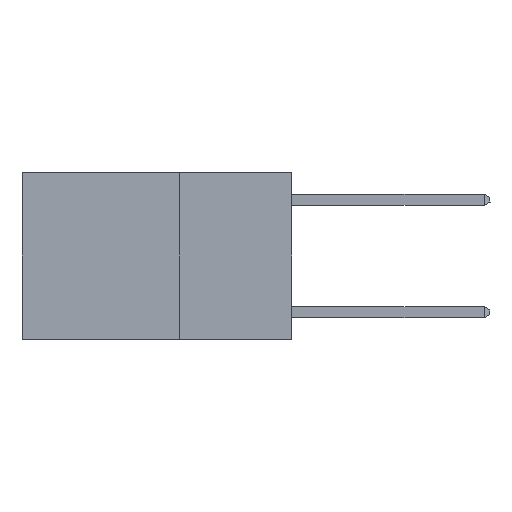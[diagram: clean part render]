
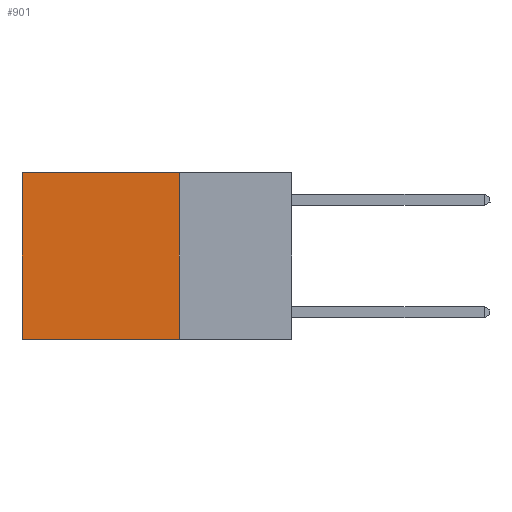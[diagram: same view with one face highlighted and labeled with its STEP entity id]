
A CAD part, left-side view. The second image highlights one B-rep face of the part: STEP entity #901.
In plain terms, the highlighted planar face has unit normal (-1, 0, 0).
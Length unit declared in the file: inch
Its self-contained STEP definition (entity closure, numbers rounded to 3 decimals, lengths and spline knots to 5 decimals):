
#151 = LINE ( 'NONE', #8592, #3359 ) ;
#761 = EDGE_CURVE ( 'NONE', #6655, #3472, #5203, .T. ) ;
#851 = DIRECTION ( 'NONE',  ( 0., 0., -1. ) ) ;
#901 = ADVANCED_FACE ( 'NONE', ( #3440 ), #1374, .F. ) ;
#1060 = CARTESIAN_POINT ( 'NONE',  ( 0.2625, 0.6, -0.37 ) ) ;
#1318 = DIRECTION ( 'NONE',  ( 0., 1., 0. ) ) ;
#1374 = PLANE ( 'NONE',  #2972 ) ;
#2316 = DIRECTION ( 'NONE',  ( 0., 0., -1. ) ) ;
#2690 = VECTOR ( 'NONE', #2316, 39.37008 ) ;
#2972 = AXIS2_PLACEMENT_3D ( 'NONE', #6697, #6428, #8793 ) ;
#3359 = VECTOR ( 'NONE', #5601, 39.37008 ) ;
#3406 = VECTOR ( 'NONE', #1318, 39.37008 ) ;
#3431 = VERTEX_POINT ( 'NONE', #4065 ) ;
#3440 = FACE_OUTER_BOUND ( 'NONE', #9101, .T. ) ;
#3472 = VERTEX_POINT ( 'NONE', #1060 ) ;
#3831 = CARTESIAN_POINT ( 'NONE',  ( 0.2625, 0.6, 0. ) ) ;
#4065 = CARTESIAN_POINT ( 'NONE',  ( 0.2625, 0.25, -0.37 ) ) ;
#4599 = CARTESIAN_POINT ( 'NONE',  ( 0.2625, 0.25, 0. ) ) ;
#5203 = LINE ( 'NONE', #3831, #8301 ) ;
#5601 = DIRECTION ( 'NONE',  ( 0., 1., 0. ) ) ;
#6103 = CARTESIAN_POINT ( 'NONE',  ( 0.2625, 0.25, 0. ) ) ;
#6174 = CARTESIAN_POINT ( 'NONE',  ( 0.2625, 0.6, 0. ) ) ;
#6318 = EDGE_CURVE ( 'NONE', #3431, #3472, #151, .T. ) ;
#6428 = DIRECTION ( 'NONE',  ( 1., 0., 0. ) ) ;
#6655 = VERTEX_POINT ( 'NONE', #6174 ) ;
#6697 = CARTESIAN_POINT ( 'NONE',  ( 0.2625, 0.25, 0. ) ) ;
#6961 = ORIENTED_EDGE ( 'NONE', *, *, #6318, .F. ) ;
#7069 = VERTEX_POINT ( 'NONE', #4599 ) ;
#7282 = CARTESIAN_POINT ( 'NONE',  ( 0.2625, 0.25, 0. ) ) ;
#7423 = LINE ( 'NONE', #7282, #3406 ) ;
#7768 = ORIENTED_EDGE ( 'NONE', *, *, #761, .T. ) ;
#7833 = EDGE_CURVE ( 'NONE', #7069, #6655, #7423, .T. ) ;
#7969 = ORIENTED_EDGE ( 'NONE', *, *, #7833, .T. ) ;
#8139 = EDGE_CURVE ( 'NONE', #7069, #3431, #9459, .T. ) ;
#8301 = VECTOR ( 'NONE', #851, 39.37008 ) ;
#8592 = CARTESIAN_POINT ( 'NONE',  ( 0.2625, 0.25, -0.37 ) ) ;
#8793 = DIRECTION ( 'NONE',  ( 0., 0., -1. ) ) ;
#9101 = EDGE_LOOP ( 'NONE', ( #7768, #6961, #9591, #7969 ) ) ;
#9459 = LINE ( 'NONE', #6103, #2690 ) ;
#9591 = ORIENTED_EDGE ( 'NONE', *, *, #8139, .F. ) ;
